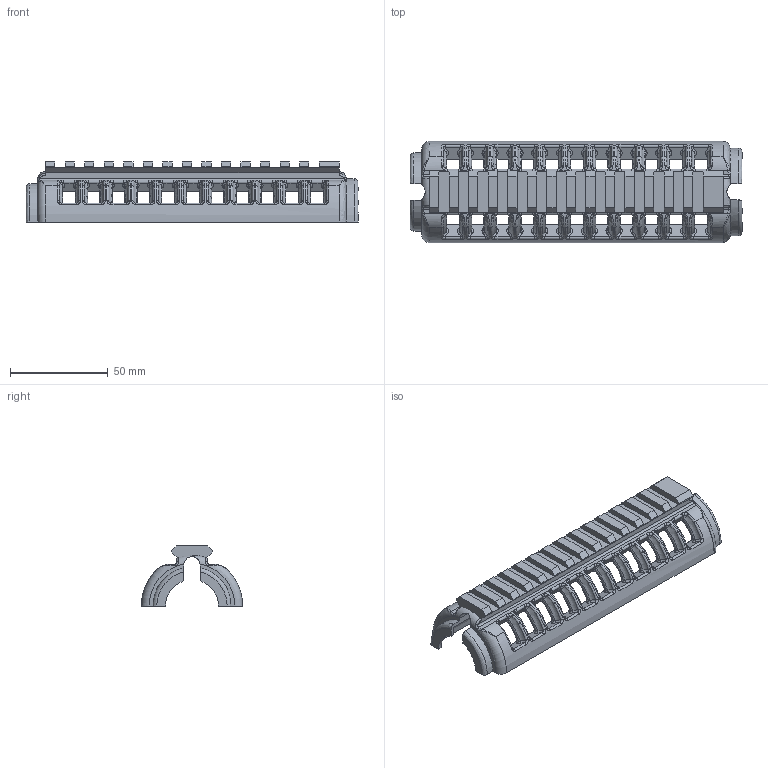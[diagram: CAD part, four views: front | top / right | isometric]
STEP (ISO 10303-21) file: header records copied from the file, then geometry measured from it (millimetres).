
FILE_DESCRIPTION (( 'STEP AP214' ), '1' );
FILE_NAME ('Carbine_Handguard_Railed.STEP', '2014-02-06T10:17:53', ( 'elpi' ), ( '' ), 'SwSTEP 2.0', 'SolidWorks 2013', '' );
FILE_SCHEMA (( 'AUTOMOTIVE_DESIGN' ));
Length unit declared in the file: inch
Products named in the file (1): Carbine_Handguard_Railed
Bounding box: 170 x 51.84 x 30.76 mm (x, y, z)
Volume: 64668.4 mm3; surface area: 34935.3 mm2
Topology: 1 solids, 1 shells, 1856 faces, 4796 edges, 2926 vertices
Faces by surface type: bspline 1058, plane 378, torus 223, cylinder 197
Entity records: 90175 total; most frequent: CARTESIAN_POINT 50372, ORIENTED_EDGE 9500, DIRECTION 5365, EDGE_CURVE 4750, VERTEX_POINT 2926, B_SPLINE_CURVE_WITH_KNOTS 2072, AXIS2_PLACEMENT_3D 2013, EDGE_LOOP 1930
